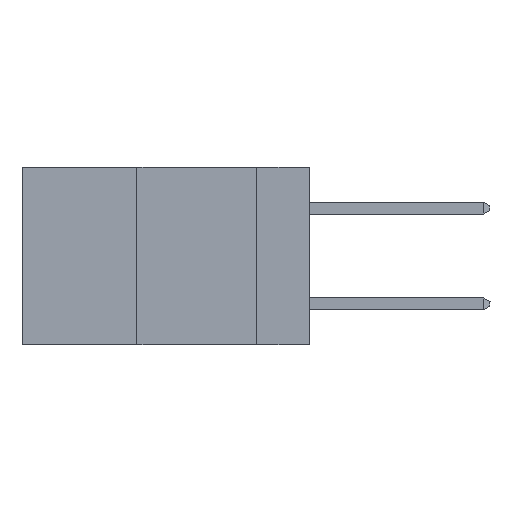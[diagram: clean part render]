
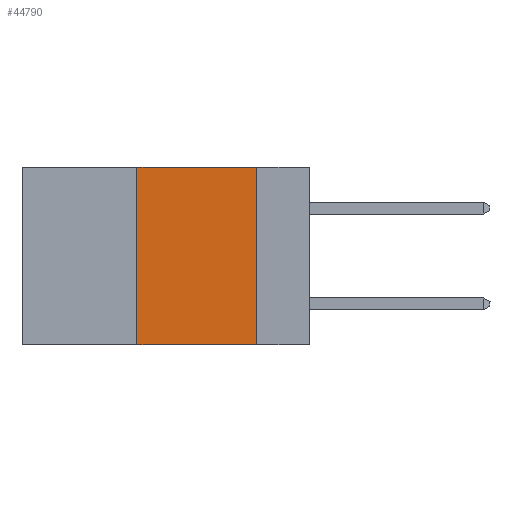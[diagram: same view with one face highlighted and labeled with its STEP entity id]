
A CAD part, left-side view. The second image highlights one B-rep face of the part: STEP entity #44790.
In plain terms, the highlighted planar face has unit normal (-1, 0, 0).
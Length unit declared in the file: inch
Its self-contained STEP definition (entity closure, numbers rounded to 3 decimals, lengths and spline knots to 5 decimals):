
#3081 = ORIENTED_EDGE ( 'NONE', *, *, #33736, .F. ) ;
#4861 = LINE ( 'NONE', #26022, #16128 ) ;
#6069 = EDGE_CURVE ( 'NONE', #36333, #31889, #39239, .T. ) ;
#7061 = CARTESIAN_POINT ( 'NONE',  ( 0., 0.36, 0. ) ) ;
#7614 = DIRECTION ( 'NONE',  ( 0., -1., 0. ) ) ;
#10471 = ORIENTED_EDGE ( 'NONE', *, *, #6069, .F. ) ;
#10991 = DIRECTION ( 'NONE',  ( 0., -1., 0. ) ) ;
#12160 = EDGE_LOOP ( 'NONE', ( #3081, #10471, #25389, #35007 ) ) ;
#16128 = VECTOR ( 'NONE', #40169, 39.37008 ) ;
#17685 = DIRECTION ( 'NONE',  ( 0., 0., -1. ) ) ;
#17871 = CARTESIAN_POINT ( 'NONE',  ( 0., 0.6, 0. ) ) ;
#21979 = CARTESIAN_POINT ( 'NONE',  ( 0., 0.11, -0.37 ) ) ;
#24973 = LINE ( 'NONE', #7061, #40149 ) ;
#25084 = CARTESIAN_POINT ( 'NONE',  ( 0., 0.36, 0. ) ) ;
#25389 = ORIENTED_EDGE ( 'NONE', *, *, #38548, .F. ) ;
#26022 = CARTESIAN_POINT ( 'NONE',  ( 0., 0.11, 0. ) ) ;
#28359 = PLANE ( 'NONE',  #35251 ) ;
#30792 = CARTESIAN_POINT ( 'NONE',  ( 0., 0.6, 0. ) ) ;
#31731 = DIRECTION ( 'NONE',  ( 0., 0., 1. ) ) ;
#31889 = VERTEX_POINT ( 'NONE', #36757 ) ;
#33224 = VERTEX_POINT ( 'NONE', #21979 ) ;
#33736 = EDGE_CURVE ( 'NONE', #31889, #33224, #4861, .T. ) ;
#34557 = VECTOR ( 'NONE', #7614, 39.37008 ) ;
#34898 = EDGE_CURVE ( 'NONE', #44841, #33224, #35626, .T. ) ;
#35007 = ORIENTED_EDGE ( 'NONE', *, *, #34898, .T. ) ;
#35251 = AXIS2_PLACEMENT_3D ( 'NONE', #30792, #41473, #17685 ) ;
#35343 = CARTESIAN_POINT ( 'NONE',  ( 0., 0.36, -0.37 ) ) ;
#35626 = LINE ( 'NONE', #42810, #45766 ) ;
#36333 = VERTEX_POINT ( 'NONE', #25084 ) ;
#36757 = CARTESIAN_POINT ( 'NONE',  ( 0., 0.11, 0. ) ) ;
#38548 = EDGE_CURVE ( 'NONE', #44841, #36333, #24973, .T. ) ;
#39239 = LINE ( 'NONE', #17871, #34557 ) ;
#40149 = VECTOR ( 'NONE', #31731, 39.37008 ) ;
#40169 = DIRECTION ( 'NONE',  ( 0., 0., -1. ) ) ;
#41473 = DIRECTION ( 'NONE',  ( 1., 0., 0. ) ) ;
#42293 = FACE_OUTER_BOUND ( 'NONE', #12160, .T. ) ;
#42810 = CARTESIAN_POINT ( 'NONE',  ( 0., 0.6, -0.37 ) ) ;
#44790 = ADVANCED_FACE ( 'NONE', ( #42293 ), #28359, .F. ) ;
#44841 = VERTEX_POINT ( 'NONE', #35343 ) ;
#45766 = VECTOR ( 'NONE', #10991, 39.37008 ) ;
